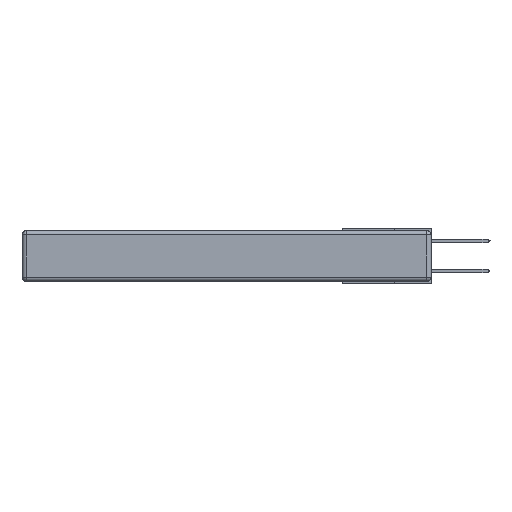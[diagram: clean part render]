
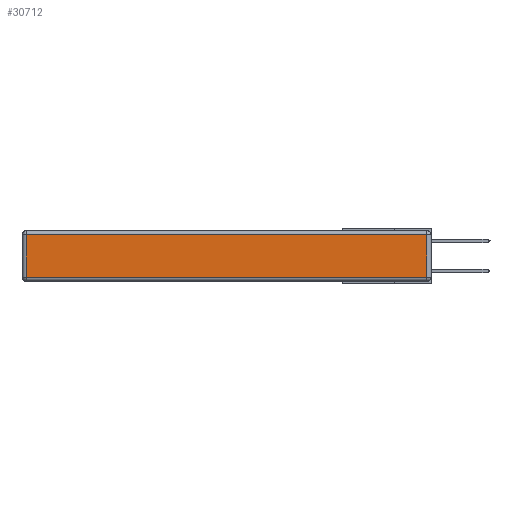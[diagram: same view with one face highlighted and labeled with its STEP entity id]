
A CAD part, left-side view. The second image highlights one B-rep face of the part: STEP entity #30712.
In plain terms, the highlighted planar face has unit normal (-1, 0, 0).
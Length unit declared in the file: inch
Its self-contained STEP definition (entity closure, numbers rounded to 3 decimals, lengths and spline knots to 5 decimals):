
#414 = ORIENTED_EDGE ( 'NONE', *, *, #9122, .T. ) ;
#3825 = AXIS2_PLACEMENT_3D ( 'NONE', #20567, #15979, #5237 ) ;
#4991 = CARTESIAN_POINT ( 'NONE',  ( 0., 0.03, -0.343 ) ) ;
#5237 = DIRECTION ( 'NONE',  ( 0., 0., 1. ) ) ;
#5880 = ORIENTED_EDGE ( 'NONE', *, *, #22919, .T. ) ;
#7366 = VERTEX_POINT ( 'NONE', #17998 ) ;
#7460 = DIRECTION ( 'NONE',  ( 0., 1., 0. ) ) ;
#8126 = CARTESIAN_POINT ( 'NONE',  ( 0., 2.72, -0.343 ) ) ;
#8491 = VECTOR ( 'NONE', #23432, 39.37008 ) ;
#8501 = ORIENTED_EDGE ( 'NONE', *, *, #27400, .T. ) ;
#9122 = EDGE_CURVE ( 'NONE', #17227, #17483, #26145, .T. ) ;
#9148 = VECTOR ( 'NONE', #15741, 39.37008 ) ;
#9330 = LINE ( 'NONE', #31220, #27195 ) ;
#11612 = VERTEX_POINT ( 'NONE', #14834 ) ;
#12017 = LINE ( 'NONE', #8126, #9148 ) ;
#12512 = ORIENTED_EDGE ( 'NONE', *, *, #25187, .T. ) ;
#13873 = CARTESIAN_POINT ( 'NONE',  ( 0., 0.03, -0.03 ) ) ;
#14834 = CARTESIAN_POINT ( 'NONE',  ( 0., 2.72, -0.03 ) ) ;
#15214 = EDGE_LOOP ( 'NONE', ( #12512, #414, #8501, #5880 ) ) ;
#15741 = DIRECTION ( 'NONE',  ( 0., 0., -1. ) ) ;
#15979 = DIRECTION ( 'NONE',  ( -1., 0., 0. ) ) ;
#16213 = LINE ( 'NONE', #32946, #24368 ) ;
#17227 = VERTEX_POINT ( 'NONE', #17553 ) ;
#17483 = VERTEX_POINT ( 'NONE', #13873 ) ;
#17553 = CARTESIAN_POINT ( 'NONE',  ( 0., 0.03, -0.313 ) ) ;
#17998 = CARTESIAN_POINT ( 'NONE',  ( 0., 2.72, -0.313 ) ) ;
#20567 = CARTESIAN_POINT ( 'NONE',  ( 0., 0., -0.343 ) ) ;
#22919 = EDGE_CURVE ( 'NONE', #11612, #7366, #12017, .T. ) ;
#23432 = DIRECTION ( 'NONE',  ( 0., 0., 1. ) ) ;
#24070 = FACE_OUTER_BOUND ( 'NONE', #15214, .T. ) ;
#24368 = VECTOR ( 'NONE', #28001, 39.37008 ) ;
#25187 = EDGE_CURVE ( 'NONE', #7366, #17227, #16213, .T. ) ;
#26145 = LINE ( 'NONE', #4991, #8491 ) ;
#27195 = VECTOR ( 'NONE', #7460, 39.37008 ) ;
#27400 = EDGE_CURVE ( 'NONE', #17483, #11612, #9330, .T. ) ;
#28001 = DIRECTION ( 'NONE',  ( 0., -1., 0. ) ) ;
#28581 = PLANE ( 'NONE',  #3825 ) ;
#30712 = ADVANCED_FACE ( 'NONE', ( #24070 ), #28581, .T. ) ;
#31220 = CARTESIAN_POINT ( 'NONE',  ( 0., 2.75, -0.03 ) ) ;
#32946 = CARTESIAN_POINT ( 'NONE',  ( 0., 0., -0.313 ) ) ;
